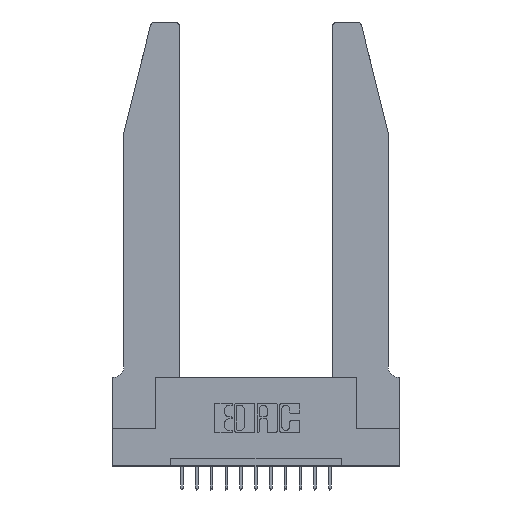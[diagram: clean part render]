
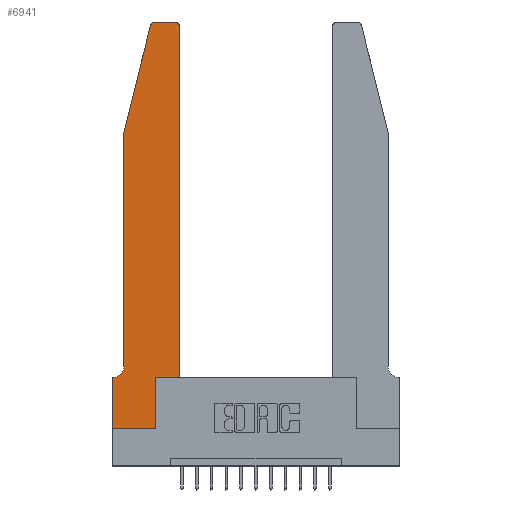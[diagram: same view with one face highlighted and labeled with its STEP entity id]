
A CAD part, top view. The second image highlights one B-rep face of the part: STEP entity #6941.
In plain terms, the highlighted planar face has unit normal (0, 0, 1).
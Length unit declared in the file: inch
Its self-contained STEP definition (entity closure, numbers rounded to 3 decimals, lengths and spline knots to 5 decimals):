
#34 = DIRECTION ( 'NONE',  ( 0., -1., 0. ) ) ;
#50 = VECTOR ( 'NONE', #3990, 39.37008 ) ;
#606 = CARTESIAN_POINT ( 'NONE',  ( 0.0055, 0.42, 0.37 ) ) ;
#621 = DIRECTION ( 'NONE',  ( 1., 0., 0. ) ) ;
#675 = FACE_OUTER_BOUND ( 'NONE', #11543, .T. ) ;
#802 = DIRECTION ( 'NONE',  ( 1., 0., 0. ) ) ;
#1110 = CARTESIAN_POINT ( 'NONE',  ( 0.0755, 0.35, 0.37 ) ) ;
#1222 = VERTEX_POINT ( 'NONE', #3595 ) ;
#1513 = CARTESIAN_POINT ( 'NONE',  ( 0., 0., 0.37 ) ) ;
#1529 = CARTESIAN_POINT ( 'NONE',  ( 0.2865, 0.35, 0.37 ) ) ;
#1689 = EDGE_CURVE ( 'NONE', #17158, #1222, #16263, .T. ) ;
#1869 = CARTESIAN_POINT ( 'NONE',  ( 0.0755, 2., 0.37 ) ) ;
#1953 = DIRECTION ( 'NONE',  ( 1., 0., 0. ) ) ;
#2221 = EDGE_CURVE ( 'NONE', #11026, #15115, #8962, .T. ) ;
#2231 = ORIENTED_EDGE ( 'NONE', *, *, #4686, .T. ) ;
#2500 = ORIENTED_EDGE ( 'NONE', *, *, #6005, .T. ) ;
#3191 = DIRECTION ( 'NONE',  ( 1., 0., 0. ) ) ;
#3327 = CARTESIAN_POINT ( 'NONE',  ( 0., 0., 0.37 ) ) ;
#3449 = CARTESIAN_POINT ( 'NONE',  ( 0.4205, 2.72, 0.37 ) ) ;
#3489 = VECTOR ( 'NONE', #14030, 39.37008 ) ;
#3494 = DIRECTION ( 'NONE',  ( -0.239, -0.971, 0. ) ) ;
#3595 = CARTESIAN_POINT ( 'NONE',  ( 0.0755, 2., 0.37 ) ) ;
#3990 = DIRECTION ( 'NONE',  ( -1., 0., 0. ) ) ;
#4283 = CARTESIAN_POINT ( 'NONE',  ( 0.4205, 2.75, 0.37 ) ) ;
#4294 = ORIENTED_EDGE ( 'NONE', *, *, #2221, .T. ) ;
#4491 = VECTOR ( 'NONE', #34, 39.37008 ) ;
#4609 = ORIENTED_EDGE ( 'NONE', *, *, #5413, .T. ) ;
#4686 = EDGE_CURVE ( 'NONE', #15368, #8366, #14724, .T. ) ;
#4751 = DIRECTION ( 'NONE',  ( 0., 0., 1. ) ) ;
#5047 = LINE ( 'NONE', #7840, #5472 ) ;
#5048 = ORIENTED_EDGE ( 'NONE', *, *, #15948, .T. ) ;
#5131 = CIRCLE ( 'NONE', #14581, 0.03 ) ;
#5413 = EDGE_CURVE ( 'NONE', #15759, #17158, #5131, .T. ) ;
#5472 = VECTOR ( 'NONE', #7431, 39.37008 ) ;
#5646 = VECTOR ( 'NONE', #3494, 39.37008 ) ;
#5790 = PLANE ( 'NONE',  #6896 ) ;
#5881 = CARTESIAN_POINT ( 'NONE',  ( 0.2605, 2.75, 0.37 ) ) ;
#6005 = EDGE_CURVE ( 'NONE', #9088, #14835, #6987, .T. ) ;
#6023 = CARTESIAN_POINT ( 'NONE',  ( 0.0755, 2., 0.37 ) ) ;
#6390 = LINE ( 'NONE', #1869, #4491 ) ;
#6424 = CARTESIAN_POINT ( 'NONE',  ( 0.0055, 0.35, 0.37 ) ) ;
#6492 = VERTEX_POINT ( 'NONE', #14166 ) ;
#6537 = DIRECTION ( 'NONE',  ( 0., 1., 0. ) ) ;
#6822 = ORIENTED_EDGE ( 'NONE', *, *, #12004, .T. ) ;
#6896 = AXIS2_PLACEMENT_3D ( 'NONE', #12571, #15093, #1953 ) ;
#6941 = ADVANCED_FACE ( 'NONE', ( #675 ), #5790, .T. ) ;
#6987 = LINE ( 'NONE', #3327, #3489 ) ;
#7047 = CIRCLE ( 'NONE', #8982, 0.07 ) ;
#7431 = DIRECTION ( 'NONE',  ( 0., 1., 0. ) ) ;
#7696 = CARTESIAN_POINT ( 'NONE',  ( 0.4505, 2.72, 0.37 ) ) ;
#7840 = CARTESIAN_POINT ( 'NONE',  ( 0.4505, 0.35, 0.37 ) ) ;
#7920 = EDGE_CURVE ( 'NONE', #8366, #8141, #13411, .T. ) ;
#7957 = EDGE_CURVE ( 'NONE', #15115, #15759, #15476, .T. ) ;
#8077 = LINE ( 'NONE', #12553, #10353 ) ;
#8141 = VERTEX_POINT ( 'NONE', #15412 ) ;
#8366 = VERTEX_POINT ( 'NONE', #1529 ) ;
#8412 = AXIS2_PLACEMENT_3D ( 'NONE', #3449, #4751, #13824 ) ;
#8750 = DIRECTION ( 'NONE',  ( -1., 0., 0. ) ) ;
#8847 = ORIENTED_EDGE ( 'NONE', *, *, #17175, .T. ) ;
#8962 = CIRCLE ( 'NONE', #8412, 0.03 ) ;
#8982 = AXIS2_PLACEMENT_3D ( 'NONE', #606, #16725, #8750 ) ;
#9088 = VERTEX_POINT ( 'NONE', #12759 ) ;
#9342 = ORIENTED_EDGE ( 'NONE', *, *, #7920, .T. ) ;
#9497 = ORIENTED_EDGE ( 'NONE', *, *, #1689, .T. ) ;
#9523 = ORIENTED_EDGE ( 'NONE', *, *, #7957, .T. ) ;
#9674 = CARTESIAN_POINT ( 'NONE',  ( 0.2865, 0., 0.37 ) ) ;
#10044 = VERTEX_POINT ( 'NONE', #6424 ) ;
#10106 = CARTESIAN_POINT ( 'NONE',  ( 0.25487, 2.72718, 0.37 ) ) ;
#10353 = VECTOR ( 'NONE', #621, 39.37008 ) ;
#11026 = VERTEX_POINT ( 'NONE', #7696 ) ;
#11160 = CARTESIAN_POINT ( 'NONE',  ( 0.284, 2.72, 0.37 ) ) ;
#11543 = EDGE_LOOP ( 'NONE', ( #9523, #4609, #9497, #6822, #15092, #5048, #2500, #12058, #2231, #9342, #8847, #4294 ) ) ;
#11949 = CARTESIAN_POINT ( 'NONE',  ( 0.2865, 0.35, 0.37 ) ) ;
#11973 = LINE ( 'NONE', #1110, #50 ) ;
#12004 = EDGE_CURVE ( 'NONE', #1222, #6492, #6390, .T. ) ;
#12058 = ORIENTED_EDGE ( 'NONE', *, *, #14194, .T. ) ;
#12261 = EDGE_CURVE ( 'NONE', #6492, #10044, #7047, .T. ) ;
#12553 = CARTESIAN_POINT ( 'NONE',  ( 0., 0., 0.37 ) ) ;
#12571 = CARTESIAN_POINT ( 'NONE',  ( 0., 0.35, 0.37 ) ) ;
#12572 = DIRECTION ( 'NONE',  ( 0., 0., 1. ) ) ;
#12759 = CARTESIAN_POINT ( 'NONE',  ( 0., 0.35, 0.37 ) ) ;
#13411 = LINE ( 'NONE', #13991, #16540 ) ;
#13824 = DIRECTION ( 'NONE',  ( 1., 0., 0. ) ) ;
#13991 = CARTESIAN_POINT ( 'NONE',  ( 0.4505, 0.35, 0.37 ) ) ;
#14030 = DIRECTION ( 'NONE',  ( 0., -1., 0. ) ) ;
#14166 = CARTESIAN_POINT ( 'NONE',  ( 0.0755, 0.42, 0.37 ) ) ;
#14194 = EDGE_CURVE ( 'NONE', #14835, #15368, #8077, .T. ) ;
#14581 = AXIS2_PLACEMENT_3D ( 'NONE', #11160, #12572, #3191 ) ;
#14724 = LINE ( 'NONE', #11949, #14932 ) ;
#14835 = VERTEX_POINT ( 'NONE', #1513 ) ;
#14932 = VECTOR ( 'NONE', #6537, 39.37008 ) ;
#15092 = ORIENTED_EDGE ( 'NONE', *, *, #12261, .T. ) ;
#15093 = DIRECTION ( 'NONE',  ( 0., 0., 1. ) ) ;
#15115 = VERTEX_POINT ( 'NONE', #4283 ) ;
#15185 = DIRECTION ( 'NONE',  ( -1., 0., 0. ) ) ;
#15368 = VERTEX_POINT ( 'NONE', #9674 ) ;
#15412 = CARTESIAN_POINT ( 'NONE',  ( 0.4505, 0.35, 0.37 ) ) ;
#15476 = LINE ( 'NONE', #5881, #17153 ) ;
#15759 = VERTEX_POINT ( 'NONE', #16189 ) ;
#15948 = EDGE_CURVE ( 'NONE', #10044, #9088, #11973, .T. ) ;
#16189 = CARTESIAN_POINT ( 'NONE',  ( 0.284, 2.75, 0.37 ) ) ;
#16263 = LINE ( 'NONE', #6023, #5646 ) ;
#16540 = VECTOR ( 'NONE', #802, 39.37008 ) ;
#16725 = DIRECTION ( 'NONE',  ( 0., 0., -1. ) ) ;
#17153 = VECTOR ( 'NONE', #15185, 39.37008 ) ;
#17158 = VERTEX_POINT ( 'NONE', #10106 ) ;
#17175 = EDGE_CURVE ( 'NONE', #8141, #11026, #5047, .T. ) ;
